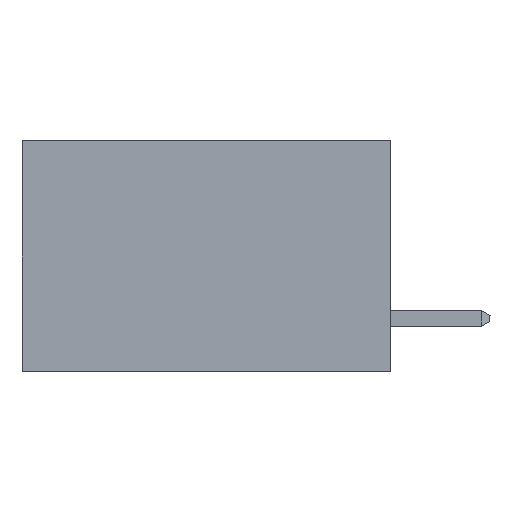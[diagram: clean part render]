
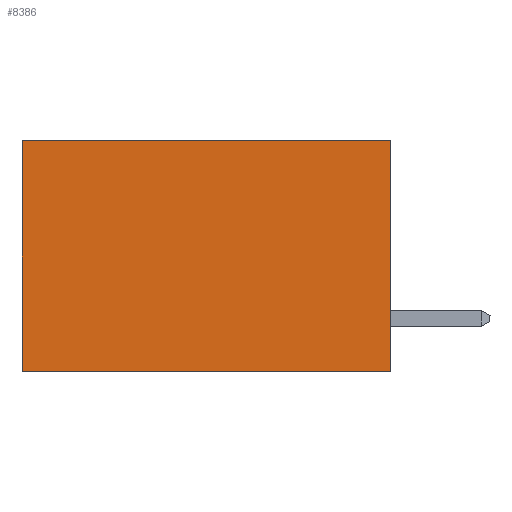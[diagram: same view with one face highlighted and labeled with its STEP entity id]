
A CAD part, left-side view. The second image highlights one B-rep face of the part: STEP entity #8386.
In plain terms, the highlighted planar face has unit normal (-1, 0, 0).
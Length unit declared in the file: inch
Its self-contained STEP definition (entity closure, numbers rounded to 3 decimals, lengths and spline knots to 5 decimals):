
#27 = DIRECTION ( 'NONE',  ( 0., 0., -1. ) ) ;
#308 = VERTEX_POINT ( 'NONE', #9650 ) ;
#500 = PLANE ( 'NONE',  #9435 ) ;
#1112 = VECTOR ( 'NONE', #27, 39.37008 ) ;
#1391 = ORIENTED_EDGE ( 'NONE', *, *, #12430, .F. ) ;
#1574 = CARTESIAN_POINT ( 'NONE',  ( 0.277, 0., -0.37 ) ) ;
#1631 = EDGE_LOOP ( 'NONE', ( #4725, #11463, #1391, #11187 ) ) ;
#1769 = CARTESIAN_POINT ( 'NONE',  ( 0.277, 0., 0. ) ) ;
#2127 = EDGE_CURVE ( 'NONE', #10446, #10809, #9772, .T. ) ;
#2585 = DIRECTION ( 'NONE',  ( 1., 0., 0. ) ) ;
#2864 = DIRECTION ( 'NONE',  ( 0., 0., -1. ) ) ;
#3084 = CARTESIAN_POINT ( 'NONE',  ( 0.277, 0., 0. ) ) ;
#3186 = CARTESIAN_POINT ( 'NONE',  ( 0.277, 0.59, -0.37 ) ) ;
#3265 = CARTESIAN_POINT ( 'NONE',  ( 0.277, 0.59, -0.37 ) ) ;
#3812 = LINE ( 'NONE', #4104, #1112 ) ;
#3814 = EDGE_CURVE ( 'NONE', #10809, #7673, #9505, .T. ) ;
#4104 = CARTESIAN_POINT ( 'NONE',  ( 0.277, 0., -0.37 ) ) ;
#4105 = VECTOR ( 'NONE', #9975, 39.37008 ) ;
#4566 = DIRECTION ( 'NONE',  ( 0., 1., 0. ) ) ;
#4725 = ORIENTED_EDGE ( 'NONE', *, *, #3814, .T. ) ;
#4910 = EDGE_CURVE ( 'NONE', #308, #7673, #6750, .T. ) ;
#6231 = CARTESIAN_POINT ( 'NONE',  ( 0.277, 0.59, 0. ) ) ;
#6333 = FACE_OUTER_BOUND ( 'NONE', #1631, .T. ) ;
#6750 = LINE ( 'NONE', #10125, #4105 ) ;
#7578 = VECTOR ( 'NONE', #2864, 39.37008 ) ;
#7673 = VERTEX_POINT ( 'NONE', #3265 ) ;
#8386 = ADVANCED_FACE ( 'NONE', ( #6333 ), #500, .F. ) ;
#9435 = AXIS2_PLACEMENT_3D ( 'NONE', #1574, #2585, #9473 ) ;
#9473 = DIRECTION ( 'NONE',  ( 0., 0., -1. ) ) ;
#9491 = VECTOR ( 'NONE', #4566, 39.37008 ) ;
#9505 = LINE ( 'NONE', #3186, #7578 ) ;
#9650 = CARTESIAN_POINT ( 'NONE',  ( 0.277, 0., -0.37 ) ) ;
#9772 = LINE ( 'NONE', #3084, #9491 ) ;
#9975 = DIRECTION ( 'NONE',  ( 0., 1., 0. ) ) ;
#10125 = CARTESIAN_POINT ( 'NONE',  ( 0.277, 0., -0.37 ) ) ;
#10446 = VERTEX_POINT ( 'NONE', #1769 ) ;
#10809 = VERTEX_POINT ( 'NONE', #6231 ) ;
#11187 = ORIENTED_EDGE ( 'NONE', *, *, #2127, .T. ) ;
#11463 = ORIENTED_EDGE ( 'NONE', *, *, #4910, .F. ) ;
#12430 = EDGE_CURVE ( 'NONE', #10446, #308, #3812, .T. ) ;
